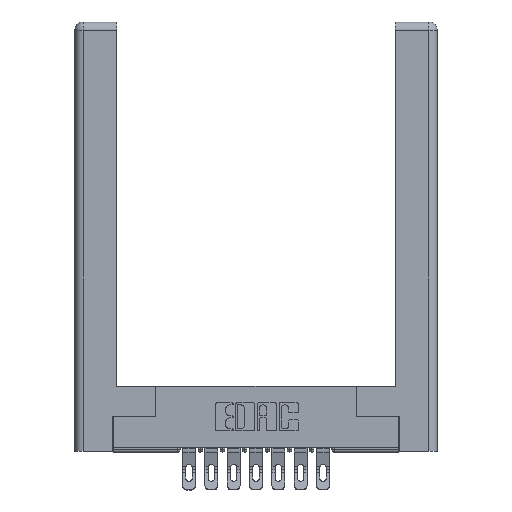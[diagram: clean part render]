
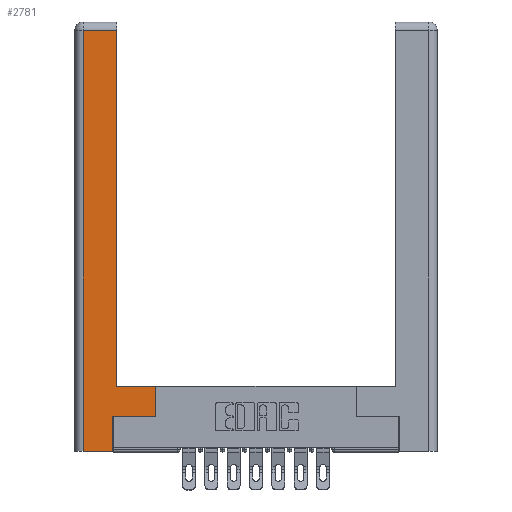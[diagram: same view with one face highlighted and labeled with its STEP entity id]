
A CAD part, top view. The second image highlights one B-rep face of the part: STEP entity #2781.
In plain terms, the highlighted planar face has unit normal (0, 0, 1).
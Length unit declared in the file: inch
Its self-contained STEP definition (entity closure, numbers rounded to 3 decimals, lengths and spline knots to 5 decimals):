
#45 = ORIENTED_EDGE ( 'NONE', *, *, #10067, .T. ) ;
#63 = LINE ( 'NONE', #5006, #4400 ) ;
#202 = CARTESIAN_POINT ( 'NONE',  ( 0.295, 0.45, 0. ) ) ;
#487 = VERTEX_POINT ( 'NONE', #1132 ) ;
#510 = LINE ( 'NONE', #5257, #1762 ) ;
#537 = ORIENTED_EDGE ( 'NONE', *, *, #5388, .T. ) ;
#907 = LINE ( 'NONE', #14979, #6361 ) ;
#984 = ORIENTED_EDGE ( 'NONE', *, *, #4261, .T. ) ;
#1071 = VECTOR ( 'NONE', #4117, 39.37008 ) ;
#1098 = CARTESIAN_POINT ( 'NONE',  ( 0.0615, 0., 0. ) ) ;
#1132 = CARTESIAN_POINT ( 'NONE',  ( 0.265, 0.245, 0. ) ) ;
#1196 = ORIENTED_EDGE ( 'NONE', *, *, #14455, .T. ) ;
#1416 = DIRECTION ( 'NONE',  ( 1., 0., 0. ) ) ;
#1762 = VECTOR ( 'NONE', #12206, 39.37008 ) ;
#1952 = CARTESIAN_POINT ( 'NONE',  ( 0.565, 0.245, 0. ) ) ;
#2188 = EDGE_CURVE ( 'NONE', #2437, #10102, #3021, .T. ) ;
#2372 = LINE ( 'NONE', #13144, #5821 ) ;
#2437 = VERTEX_POINT ( 'NONE', #12782 ) ;
#2781 = ADVANCED_FACE ( 'NONE', ( #2822 ), #13620, .F. ) ;
#2822 = FACE_OUTER_BOUND ( 'NONE', #3446, .T. ) ;
#3021 = LINE ( 'NONE', #14157, #15095 ) ;
#3215 = CARTESIAN_POINT ( 'NONE',  ( 0.565, 0.45, 0. ) ) ;
#3446 = EDGE_LOOP ( 'NONE', ( #984, #6464, #10639, #537, #45, #1196, #5684, #5409 ) ) ;
#3484 = VERTEX_POINT ( 'NONE', #3215 ) ;
#3828 = DIRECTION ( 'NONE',  ( 0., 1., 0. ) ) ;
#4086 = LINE ( 'NONE', #14610, #7544 ) ;
#4117 = DIRECTION ( 'NONE',  ( 1., 0., 0. ) ) ;
#4187 = CARTESIAN_POINT ( 'NONE',  ( 0.295, 2.94, 0. ) ) ;
#4261 = EDGE_CURVE ( 'NONE', #11232, #8936, #63, .T. ) ;
#4400 = VECTOR ( 'NONE', #3828, 39.37008 ) ;
#5006 = CARTESIAN_POINT ( 'NONE',  ( 0.295, 3., 0. ) ) ;
#5257 = CARTESIAN_POINT ( 'NONE',  ( 0.565, 0.45, 0. ) ) ;
#5388 = EDGE_CURVE ( 'NONE', #10102, #8106, #2372, .T. ) ;
#5409 = ORIENTED_EDGE ( 'NONE', *, *, #14755, .T. ) ;
#5684 = ORIENTED_EDGE ( 'NONE', *, *, #14777, .T. ) ;
#5821 = VECTOR ( 'NONE', #1416, 39.37008 ) ;
#6171 = EDGE_CURVE ( 'NONE', #8936, #2437, #4086, .T. ) ;
#6361 = VECTOR ( 'NONE', #9198, 39.37008 ) ;
#6464 = ORIENTED_EDGE ( 'NONE', *, *, #6171, .T. ) ;
#7041 = CARTESIAN_POINT ( 'NONE',  ( 0.295, 0.45, 0. ) ) ;
#7258 = DIRECTION ( 'NONE',  ( -1., 0., 0. ) ) ;
#7544 = VECTOR ( 'NONE', #13409, 39.37008 ) ;
#8106 = VERTEX_POINT ( 'NONE', #14049 ) ;
#8503 = VECTOR ( 'NONE', #7258, 39.37008 ) ;
#8910 = CARTESIAN_POINT ( 'NONE',  ( 0., 0., 0. ) ) ;
#8936 = VERTEX_POINT ( 'NONE', #4187 ) ;
#9198 = DIRECTION ( 'NONE',  ( 0., 1., 0. ) ) ;
#9278 = LINE ( 'NONE', #1952, #1071 ) ;
#10041 = DIRECTION ( 'NONE',  ( -1., 0., 0. ) ) ;
#10067 = EDGE_CURVE ( 'NONE', #8106, #487, #907, .T. ) ;
#10102 = VERTEX_POINT ( 'NONE', #1098 ) ;
#10178 = DIRECTION ( 'NONE',  ( 0., 0., -1. ) ) ;
#10325 = AXIS2_PLACEMENT_3D ( 'NONE', #8910, #10178, #10041 ) ;
#10639 = ORIENTED_EDGE ( 'NONE', *, *, #2188, .T. ) ;
#11232 = VERTEX_POINT ( 'NONE', #7041 ) ;
#11832 = DIRECTION ( 'NONE',  ( 0., -1., 0. ) ) ;
#12118 = VERTEX_POINT ( 'NONE', #13915 ) ;
#12206 = DIRECTION ( 'NONE',  ( 0., 1., 0. ) ) ;
#12782 = CARTESIAN_POINT ( 'NONE',  ( 0.0615, 2.94, 0. ) ) ;
#13144 = CARTESIAN_POINT ( 'NONE',  ( 0.265, 0., 0. ) ) ;
#13409 = DIRECTION ( 'NONE',  ( -1., 0., 0. ) ) ;
#13620 = PLANE ( 'NONE',  #10325 ) ;
#13915 = CARTESIAN_POINT ( 'NONE',  ( 0.565, 0.245, 0. ) ) ;
#14049 = CARTESIAN_POINT ( 'NONE',  ( 0.265, 0., 0. ) ) ;
#14157 = CARTESIAN_POINT ( 'NONE',  ( 0.0615, 0., 0. ) ) ;
#14455 = EDGE_CURVE ( 'NONE', #487, #12118, #9278, .T. ) ;
#14610 = CARTESIAN_POINT ( 'NONE',  ( 0.0615, 2.94, 0. ) ) ;
#14755 = EDGE_CURVE ( 'NONE', #3484, #11232, #14756, .T. ) ;
#14756 = LINE ( 'NONE', #202, #8503 ) ;
#14777 = EDGE_CURVE ( 'NONE', #12118, #3484, #510, .T. ) ;
#14979 = CARTESIAN_POINT ( 'NONE',  ( 0.265, 0.245, 0. ) ) ;
#15095 = VECTOR ( 'NONE', #11832, 39.37008 ) ;
